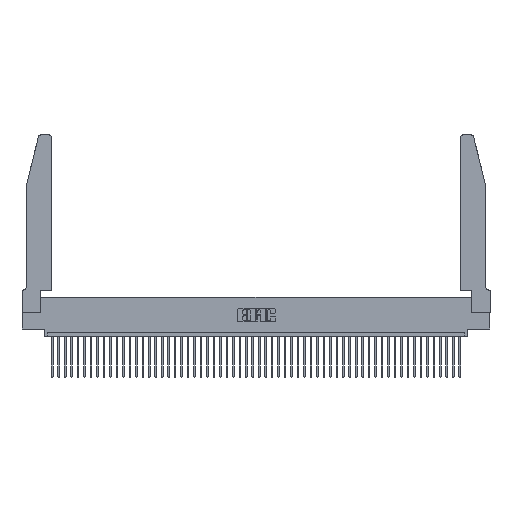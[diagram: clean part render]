
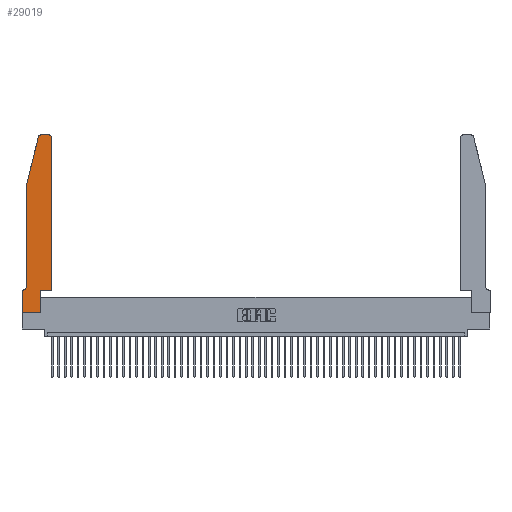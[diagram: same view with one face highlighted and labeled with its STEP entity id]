
A CAD part, top view. The second image highlights one B-rep face of the part: STEP entity #29019.
In plain terms, the highlighted planar face has unit normal (0, 0, 1).
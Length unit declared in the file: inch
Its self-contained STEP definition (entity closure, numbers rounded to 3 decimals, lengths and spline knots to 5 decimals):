
#68 = VECTOR ( 'NONE', #47567, 39.37008 ) ;
#431 = ORIENTED_EDGE ( 'NONE', *, *, #9918, .T. ) ;
#1282 = VECTOR ( 'NONE', #35028, 39.37008 ) ;
#1432 = LINE ( 'NONE', #42350, #40188 ) ;
#1517 = AXIS2_PLACEMENT_3D ( 'NONE', #25068, #44133, #1827 ) ;
#1827 = DIRECTION ( 'NONE',  ( 1., 0., 0. ) ) ;
#2083 = CARTESIAN_POINT ( 'NONE',  ( 0.2865, 0.35, 0.37 ) ) ;
#2085 = DIRECTION ( 'NONE',  ( 1., 0., 0. ) ) ;
#3232 = ORIENTED_EDGE ( 'NONE', *, *, #9733, .T. ) ;
#3809 = ORIENTED_EDGE ( 'NONE', *, *, #46630, .T. ) ;
#4452 = CARTESIAN_POINT ( 'NONE',  ( 0.0755, 2., 0.37 ) ) ;
#5412 = EDGE_LOOP ( 'NONE', ( #7990, #431, #45012, #48749, #43728, #7692, #11270, #3232, #48632, #3809, #25661, #29041 ) ) ;
#5602 = DIRECTION ( 'NONE',  ( -1., 0., 0. ) ) ;
#7692 = ORIENTED_EDGE ( 'NONE', *, *, #42234, .T. ) ;
#7990 = ORIENTED_EDGE ( 'NONE', *, *, #28142, .T. ) ;
#8116 = EDGE_CURVE ( 'NONE', #21600, #31761, #11848, .T. ) ;
#8798 = LINE ( 'NONE', #35069, #38497 ) ;
#9184 = LINE ( 'NONE', #11730, #13407 ) ;
#9733 = EDGE_CURVE ( 'NONE', #45823, #47871, #37305, .T. ) ;
#9741 = CARTESIAN_POINT ( 'NONE',  ( 0.25487, 2.72718, 0.37 ) ) ;
#9826 = LINE ( 'NONE', #40262, #46745 ) ;
#9918 = EDGE_CURVE ( 'NONE', #16621, #20502, #16047, .T. ) ;
#10401 = CARTESIAN_POINT ( 'NONE',  ( 0., 0., 0.37 ) ) ;
#11270 = ORIENTED_EDGE ( 'NONE', *, *, #42868, .T. ) ;
#11569 = DIRECTION ( 'NONE',  ( 0., 1., 0. ) ) ;
#11730 = CARTESIAN_POINT ( 'NONE',  ( 0.4505, 0.35, 0.37 ) ) ;
#11848 = CIRCLE ( 'NONE', #42421, 0.07 ) ;
#13407 = VECTOR ( 'NONE', #11569, 39.37008 ) ;
#13988 = LINE ( 'NONE', #40145, #68 ) ;
#14548 = VERTEX_POINT ( 'NONE', #17718 ) ;
#14941 = AXIS2_PLACEMENT_3D ( 'NONE', #48919, #33610, #2085 ) ;
#16047 = CIRCLE ( 'NONE', #14941, 0.03 ) ;
#16621 = VERTEX_POINT ( 'NONE', #18513 ) ;
#17021 = VERTEX_POINT ( 'NONE', #2083 ) ;
#17210 = DIRECTION ( 'NONE',  ( -1., 0., 0. ) ) ;
#17522 = DIRECTION ( 'NONE',  ( 1., 0., 0. ) ) ;
#17718 = CARTESIAN_POINT ( 'NONE',  ( 0.4505, 2.72, 0.37 ) ) ;
#18513 = CARTESIAN_POINT ( 'NONE',  ( 0.284, 2.75, 0.37 ) ) ;
#18604 = VERTEX_POINT ( 'NONE', #19734 ) ;
#19734 = CARTESIAN_POINT ( 'NONE',  ( 0., 0.35, 0.37 ) ) ;
#20502 = VERTEX_POINT ( 'NONE', #9741 ) ;
#20732 = FACE_OUTER_BOUND ( 'NONE', #5412, .T. ) ;
#20882 = VERTEX_POINT ( 'NONE', #35129 ) ;
#21600 = VERTEX_POINT ( 'NONE', #36422 ) ;
#23106 = LINE ( 'NONE', #4452, #40019 ) ;
#23421 = VECTOR ( 'NONE', #43060, 39.37008 ) ;
#23932 = EDGE_CURVE ( 'NONE', #20502, #35817, #23106, .T. ) ;
#24018 = CARTESIAN_POINT ( 'NONE',  ( 0.4205, 2.72, 0.37 ) ) ;
#24032 = LINE ( 'NONE', #31302, #23421 ) ;
#25068 = CARTESIAN_POINT ( 'NONE',  ( 0., 0.35, 0.37 ) ) ;
#25661 = ORIENTED_EDGE ( 'NONE', *, *, #38419, .T. ) ;
#25723 = CARTESIAN_POINT ( 'NONE',  ( 0.0755, 2., 0.37 ) ) ;
#27029 = VECTOR ( 'NONE', #17522, 39.37008 ) ;
#28142 = EDGE_CURVE ( 'NONE', #20882, #16621, #1432, .T. ) ;
#28360 = CARTESIAN_POINT ( 'NONE',  ( 0.0055, 0.42, 0.37 ) ) ;
#29019 = ADVANCED_FACE ( 'NONE', ( #20732 ), #36591, .T. ) ;
#29041 = ORIENTED_EDGE ( 'NONE', *, *, #34155, .T. ) ;
#31302 = CARTESIAN_POINT ( 'NONE',  ( 0.0755, 2., 0.37 ) ) ;
#31740 = CARTESIAN_POINT ( 'NONE',  ( 0.2865, 0., 0.37 ) ) ;
#31761 = VERTEX_POINT ( 'NONE', #37057 ) ;
#32585 = DIRECTION ( 'NONE',  ( 0., 0., -1. ) ) ;
#33610 = DIRECTION ( 'NONE',  ( 0., 0., 1. ) ) ;
#34155 = EDGE_CURVE ( 'NONE', #14548, #20882, #46855, .T. ) ;
#34791 = DIRECTION ( 'NONE',  ( -1., 0., 0. ) ) ;
#35028 = DIRECTION ( 'NONE',  ( 0., 1., 0. ) ) ;
#35069 = CARTESIAN_POINT ( 'NONE',  ( 0.4505, 0.35, 0.37 ) ) ;
#35129 = CARTESIAN_POINT ( 'NONE',  ( 0.4205, 2.75, 0.37 ) ) ;
#35817 = VERTEX_POINT ( 'NONE', #25723 ) ;
#35837 = LINE ( 'NONE', #39061, #1282 ) ;
#35872 = DIRECTION ( 'NONE',  ( 0., 0., 1. ) ) ;
#35968 = CARTESIAN_POINT ( 'NONE',  ( 0.4505, 0.35, 0.37 ) ) ;
#36422 = CARTESIAN_POINT ( 'NONE',  ( 0.0755, 0.42, 0.37 ) ) ;
#36591 = PLANE ( 'NONE',  #1517 ) ;
#36876 = CARTESIAN_POINT ( 'NONE',  ( 0., 0., 0.37 ) ) ;
#37057 = CARTESIAN_POINT ( 'NONE',  ( 0.0055, 0.35, 0.37 ) ) ;
#37305 = LINE ( 'NONE', #36876, #27029 ) ;
#38419 = EDGE_CURVE ( 'NONE', #47814, #14548, #9184, .T. ) ;
#38497 = VECTOR ( 'NONE', #42774, 39.37008 ) ;
#38679 = AXIS2_PLACEMENT_3D ( 'NONE', #24018, #35872, #43084 ) ;
#39061 = CARTESIAN_POINT ( 'NONE',  ( 0.2865, 0.35, 0.37 ) ) ;
#40019 = VECTOR ( 'NONE', #46917, 39.37008 ) ;
#40145 = CARTESIAN_POINT ( 'NONE',  ( 0., 0., 0.37 ) ) ;
#40188 = VECTOR ( 'NONE', #34791, 39.37008 ) ;
#40262 = CARTESIAN_POINT ( 'NONE',  ( 0.0755, 0.35, 0.37 ) ) ;
#40652 = EDGE_CURVE ( 'NONE', #47871, #17021, #35837, .T. ) ;
#42234 = EDGE_CURVE ( 'NONE', #31761, #18604, #9826, .T. ) ;
#42350 = CARTESIAN_POINT ( 'NONE',  ( 0.2605, 2.75, 0.37 ) ) ;
#42421 = AXIS2_PLACEMENT_3D ( 'NONE', #28360, #32585, #5602 ) ;
#42774 = DIRECTION ( 'NONE',  ( 1., 0., 0. ) ) ;
#42868 = EDGE_CURVE ( 'NONE', #18604, #45823, #13988, .T. ) ;
#43060 = DIRECTION ( 'NONE',  ( 0., -1., 0. ) ) ;
#43084 = DIRECTION ( 'NONE',  ( 1., 0., 0. ) ) ;
#43728 = ORIENTED_EDGE ( 'NONE', *, *, #8116, .T. ) ;
#44133 = DIRECTION ( 'NONE',  ( 0., 0., 1. ) ) ;
#45012 = ORIENTED_EDGE ( 'NONE', *, *, #23932, .T. ) ;
#45380 = EDGE_CURVE ( 'NONE', #35817, #21600, #24032, .T. ) ;
#45823 = VERTEX_POINT ( 'NONE', #10401 ) ;
#46630 = EDGE_CURVE ( 'NONE', #17021, #47814, #8798, .T. ) ;
#46745 = VECTOR ( 'NONE', #17210, 39.37008 ) ;
#46855 = CIRCLE ( 'NONE', #38679, 0.03 ) ;
#46917 = DIRECTION ( 'NONE',  ( -0.239, -0.971, 0. ) ) ;
#47567 = DIRECTION ( 'NONE',  ( 0., -1., 0. ) ) ;
#47814 = VERTEX_POINT ( 'NONE', #35968 ) ;
#47871 = VERTEX_POINT ( 'NONE', #31740 ) ;
#48632 = ORIENTED_EDGE ( 'NONE', *, *, #40652, .T. ) ;
#48749 = ORIENTED_EDGE ( 'NONE', *, *, #45380, .T. ) ;
#48919 = CARTESIAN_POINT ( 'NONE',  ( 0.284, 2.72, 0.37 ) ) ;
